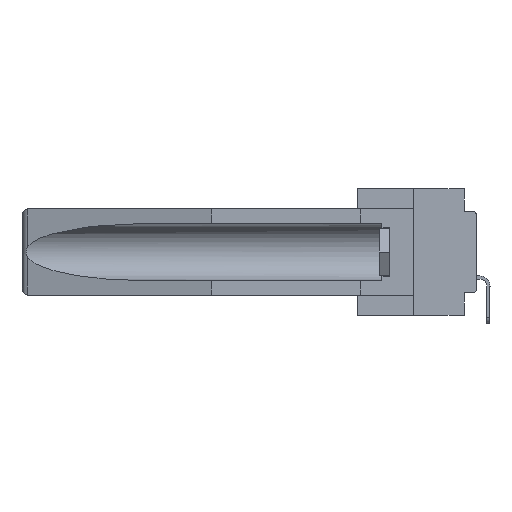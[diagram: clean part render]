
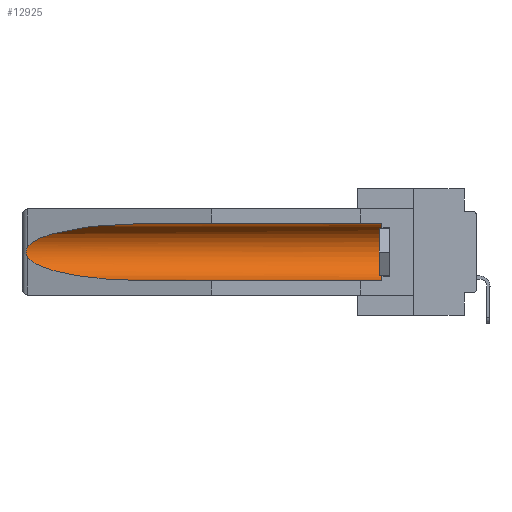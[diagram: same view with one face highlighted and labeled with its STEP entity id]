
A CAD part, left-side view. The second image highlights one B-rep face of the part: STEP entity #12925.
In plain terms, the highlighted cylindrical face has radius 2.857 mm (diameter 5.715 mm), a partial arc.
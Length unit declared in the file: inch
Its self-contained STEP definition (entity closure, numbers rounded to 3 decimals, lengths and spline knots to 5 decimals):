
#685 = CIRCLE ( 'NONE', #37463, 0.1125 ) ;
#1444 = CARTESIAN_POINT ( 'NONE',  ( 0.155, -0.30754, -0.1715 ) ) ;
#1504 = CARTESIAN_POINT ( 'NONE',  ( 0.155, 0.126, -0.284 ) ) ;
#1775 = CARTESIAN_POINT ( 'NONE',  ( 0.26537, 1.52718, -0.14972 ) ) ;
#4682 = CARTESIAN_POINT ( 'NONE',  ( 0.155, 0.126, -0.059 ) ) ;
#4913 = CARTESIAN_POINT ( 'NONE',  ( 0.155, 1.07973, -0.059 ) ) ;
#4943 = CYLINDRICAL_SURFACE ( 'NONE', #19072, 0.1125 ) ;
#5601 = CARTESIAN_POINT ( 'NONE',  ( 0.26597, 1.5296, -0.19026 ) ) ;
#8039 = EDGE_CURVE ( 'NONE', #30259, #25298, #14656, .T. ) ;
#8368 = ORIENTED_EDGE ( 'NONE', *, *, #13867, .T. ) ;
#8729 = CARTESIAN_POINT ( 'NONE',  ( 0.155, 1.07973, -0.059 ) ) ;
#8733 = EDGE_LOOP ( 'NONE', ( #8368, #32401, #11323, #33081, #17434, #26978 ) ) ;
#8737 = CARTESIAN_POINT ( 'NONE',  ( 0.26597, 1.52961, -0.15275 ) ) ;
#10760 = CARTESIAN_POINT ( 'NONE',  ( 0.2673, 1.5327, -0.16383 ) ) ;
#10983 = CARTESIAN_POINT ( 'NONE',  ( 0.25451, 1.48313, -0.09465 ) ) ;
#11013 = LINE ( 'NONE', #21698, #37709 ) ;
#11210 = CARTESIAN_POINT ( 'NONE',  ( 0.25451, 1.48313, -0.24835 ) ) ;
#11323 = ORIENTED_EDGE ( 'NONE', *, *, #36532, .T. ) ;
#11673 = CARTESIAN_POINT ( 'NONE',  ( 0.26654, 1.53092, -0.15636 ) ) ;
#11756 = B_SPLINE_CURVE_WITH_KNOTS ( 'NONE', 3,
 ( #1775, #8737, #11673, #10760, #26465, #14787, #34531, #17706, #5601, #13886 ),
 .UNSPECIFIED., .F., .F.,
 ( 4, 2, 2, 2, 4 ),
 ( 0., 0.00029, 0.00058, 0.00087, 0.00117 ),
 .UNSPECIFIED. ) ;
#12925 = ADVANCED_FACE ( 'NONE', ( #37338 ), #4943, .F. ) ;
#13305 = VECTOR ( 'NONE', #19907, 39.37008 ) ;
#13867 = EDGE_CURVE ( 'NONE', #14717, #24918, #38037, .T. ) ;
#13886 = CARTESIAN_POINT ( 'NONE',  ( 0.26537, 1.52718, -0.19328 ) ) ;
#14140 = CARTESIAN_POINT ( 'NONE',  ( 0.21114, 1.30732, -0.284 ) ) ;
#14656 = LINE ( 'NONE', #31792, #13305 ) ;
#14717 = VERTEX_POINT ( 'NONE', #8729 ) ;
#14771 = DIRECTION ( 'NONE',  ( 0., -1., 0. ) ) ;
#14787 = CARTESIAN_POINT ( 'NONE',  ( 0.2675, 1.53308, -0.17534 ) ) ;
#15485 = VERTEX_POINT ( 'NONE', #4682 ) ;
#17434 = ORIENTED_EDGE ( 'NONE', *, *, #31724, .T. ) ;
#17706 = CARTESIAN_POINT ( 'NONE',  ( 0.26655, 1.53094, -0.18657 ) ) ;
#18200 = DIRECTION ( 'NONE',  ( 0., 1., 0. ) ) ;
#19072 = AXIS2_PLACEMENT_3D ( 'NONE', #1444, #33821, #37137 ) ;
#19907 = DIRECTION ( 'NONE',  ( 0., 1., 0. ) ) ;
#20355 = CARTESIAN_POINT ( 'NONE',  ( 0.155, 1.07973, -0.284 ) ) ;
#21698 = CARTESIAN_POINT ( 'NONE',  ( 0.155, -0.30754, -0.059 ) ) ;
#22859 = CARTESIAN_POINT ( 'NONE',  ( 0.26537, 1.52718, -0.14972 ) ) ;
#22964 = DIRECTION ( 'NONE',  ( 0., 0., 1. ) ) ;
#24918 = VERTEX_POINT ( 'NONE', #27944 ) ;
#25249 = VERTEX_POINT ( 'NONE', #37791 ) ;
#25298 = VERTEX_POINT ( 'NONE', #37597 ) ;
#25387 =( BOUNDED_CURVE ( )  B_SPLINE_CURVE ( 3, ( #32042, #11210, #14140, #20355 ),
 .UNSPECIFIED., .F., .F. ) 
 B_SPLINE_CURVE_WITH_KNOTS ( ( 4, 4 ),
 ( 0.1948, 1.5708 ),
 .UNSPECIFIED. ) 
 CURVE ( )  GEOMETRIC_REPRESENTATION_ITEM ( )  RATIONAL_B_SPLINE_CURVE ( ( 1., 0.848, 0.848, 1. ) ) 
 REPRESENTATION_ITEM ( '' )  );
#25394 = EDGE_CURVE ( 'NONE', #24918, #25249, #11756, .T. ) ;
#26465 = CARTESIAN_POINT ( 'NONE',  ( 0.2675, 1.53308, -0.16763 ) ) ;
#26978 = ORIENTED_EDGE ( 'NONE', *, *, #36629, .T. ) ;
#27944 = CARTESIAN_POINT ( 'NONE',  ( 0.26537, 1.52718, -0.14972 ) ) ;
#28717 = CARTESIAN_POINT ( 'NONE',  ( 0.21114, 1.30732, -0.059 ) ) ;
#29199 = CARTESIAN_POINT ( 'NONE',  ( 0.155, 0.126, -0.1715 ) ) ;
#30259 = VERTEX_POINT ( 'NONE', #1504 ) ;
#31724 = EDGE_CURVE ( 'NONE', #30259, #15485, #685, .T. ) ;
#31792 = CARTESIAN_POINT ( 'NONE',  ( 0.155, -0.30754, -0.284 ) ) ;
#32042 = CARTESIAN_POINT ( 'NONE',  ( 0.26537, 1.52718, -0.19328 ) ) ;
#32401 = ORIENTED_EDGE ( 'NONE', *, *, #25394, .T. ) ;
#33081 = ORIENTED_EDGE ( 'NONE', *, *, #8039, .F. ) ;
#33821 = DIRECTION ( 'NONE',  ( 0., 1., 0. ) ) ;
#34531 = CARTESIAN_POINT ( 'NONE',  ( 0.2673, 1.53269, -0.17917 ) ) ;
#36532 = EDGE_CURVE ( 'NONE', #25249, #25298, #25387, .T. ) ;
#36629 = EDGE_CURVE ( 'NONE', #15485, #14717, #11013, .T. ) ;
#37137 = DIRECTION ( 'NONE',  ( 0., 0., 1. ) ) ;
#37338 = FACE_OUTER_BOUND ( 'NONE', #8733, .T. ) ;
#37463 = AXIS2_PLACEMENT_3D ( 'NONE', #29199, #14771, #22964 ) ;
#37597 = CARTESIAN_POINT ( 'NONE',  ( 0.155, 1.07973, -0.284 ) ) ;
#37709 = VECTOR ( 'NONE', #18200, 39.37008 ) ;
#37791 = CARTESIAN_POINT ( 'NONE',  ( 0.26537, 1.52718, -0.19328 ) ) ;
#38037 =( BOUNDED_CURVE ( )  B_SPLINE_CURVE ( 3, ( #4913, #28717, #10983, #22859 ),
 .UNSPECIFIED., .F., .F. ) 
 B_SPLINE_CURVE_WITH_KNOTS ( ( 4, 4 ),
 ( 4.71239, 6.08839 ),
 .UNSPECIFIED. ) 
 CURVE ( )  GEOMETRIC_REPRESENTATION_ITEM ( )  RATIONAL_B_SPLINE_CURVE ( ( 1., 0.848, 0.848, 1. ) ) 
 REPRESENTATION_ITEM ( '' )  );
